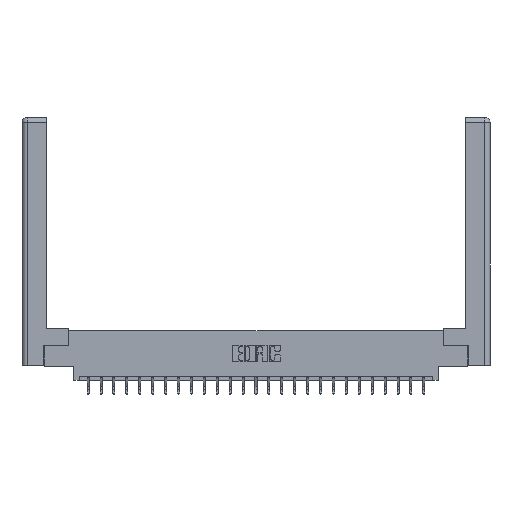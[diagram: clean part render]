
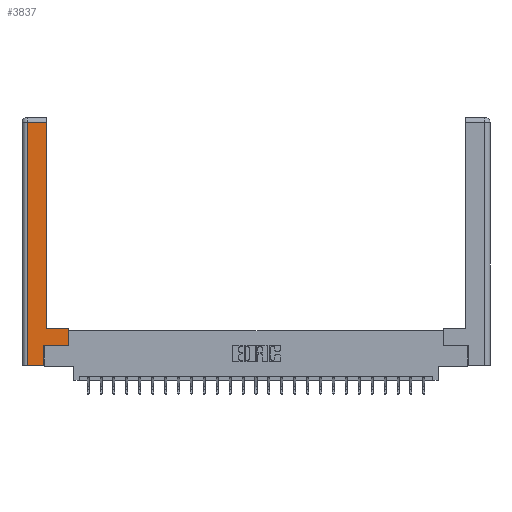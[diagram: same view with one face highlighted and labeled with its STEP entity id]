
A CAD part, top view. The second image highlights one B-rep face of the part: STEP entity #3837.
In plain terms, the highlighted planar face has unit normal (0, 0, 1).
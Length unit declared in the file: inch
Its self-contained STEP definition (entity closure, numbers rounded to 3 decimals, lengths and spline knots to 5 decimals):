
#94 = CARTESIAN_POINT ( 'NONE',  ( 0.295, 0.45, 0. ) ) ;
#168 = EDGE_LOOP ( 'NONE', ( #11904, #22617, #9253, #5354, #22514, #23321, #8111, #20060 ) ) ;
#1802 = CARTESIAN_POINT ( 'NONE',  ( 0.0615, 0., 0. ) ) ;
#2093 = FACE_OUTER_BOUND ( 'NONE', #168, .T. ) ;
#2310 = DIRECTION ( 'NONE',  ( 0., -1., 0. ) ) ;
#2415 = DIRECTION ( 'NONE',  ( 0., 1., 0. ) ) ;
#2947 = LINE ( 'NONE', #94, #7948 ) ;
#2972 = VECTOR ( 'NONE', #21944, 39.37008 ) ;
#3542 = VERTEX_POINT ( 'NONE', #5979 ) ;
#3837 = ADVANCED_FACE ( 'NONE', ( #2093 ), #12183, .F. ) ;
#4203 = LINE ( 'NONE', #12570, #6073 ) ;
#4324 = LINE ( 'NONE', #15668, #4620 ) ;
#4620 = VECTOR ( 'NONE', #9841, 39.37008 ) ;
#5225 = LINE ( 'NONE', #15964, #25583 ) ;
#5354 = ORIENTED_EDGE ( 'NONE', *, *, #21883, .T. ) ;
#5979 = CARTESIAN_POINT ( 'NONE',  ( 0.565, 0.45, 0. ) ) ;
#6031 = EDGE_CURVE ( 'NONE', #15035, #3542, #18403, .T. ) ;
#6073 = VECTOR ( 'NONE', #25053, 39.37008 ) ;
#6097 = DIRECTION ( 'NONE',  ( 0., 0., -1. ) ) ;
#6559 = CARTESIAN_POINT ( 'NONE',  ( 0.0615, 2.94, 0. ) ) ;
#7174 = VECTOR ( 'NONE', #2310, 39.37008 ) ;
#7285 = CARTESIAN_POINT ( 'NONE',  ( 0.295, 0.45, 0. ) ) ;
#7483 = CARTESIAN_POINT ( 'NONE',  ( 0.295, 2.94, 0. ) ) ;
#7785 = CARTESIAN_POINT ( 'NONE',  ( 0.565, 0.245, 0. ) ) ;
#7948 = VECTOR ( 'NONE', #22018, 39.37008 ) ;
#8111 = ORIENTED_EDGE ( 'NONE', *, *, #6031, .T. ) ;
#8415 = DIRECTION ( 'NONE',  ( -1., 0., 0. ) ) ;
#9169 = EDGE_CURVE ( 'NONE', #3542, #12504, #2947, .T. ) ;
#9253 = ORIENTED_EDGE ( 'NONE', *, *, #20976, .T. ) ;
#9328 = VECTOR ( 'NONE', #2415, 39.37008 ) ;
#9619 = CARTESIAN_POINT ( 'NONE',  ( 0.0615, 2.94, 0. ) ) ;
#9841 = DIRECTION ( 'NONE',  ( 0., 1., 0. ) ) ;
#10779 = CARTESIAN_POINT ( 'NONE',  ( 0.265, 0.245, 0. ) ) ;
#11264 = VECTOR ( 'NONE', #15727, 39.37008 ) ;
#11442 = CARTESIAN_POINT ( 'NONE',  ( 0.565, 0.245, 0. ) ) ;
#11863 = EDGE_CURVE ( 'NONE', #19201, #24317, #17455, .T. ) ;
#11904 = ORIENTED_EDGE ( 'NONE', *, *, #16731, .T. ) ;
#12183 = PLANE ( 'NONE',  #22511 ) ;
#12315 = CARTESIAN_POINT ( 'NONE',  ( 0.565, 0.45, 0. ) ) ;
#12369 = CARTESIAN_POINT ( 'NONE',  ( 0., 0., 0. ) ) ;
#12504 = VERTEX_POINT ( 'NONE', #7285 ) ;
#12570 = CARTESIAN_POINT ( 'NONE',  ( 0.295, 3., 0. ) ) ;
#14112 = EDGE_CURVE ( 'NONE', #19523, #18024, #4324, .T. ) ;
#15035 = VERTEX_POINT ( 'NONE', #11442 ) ;
#15098 = CARTESIAN_POINT ( 'NONE',  ( 0.265, 0., 0. ) ) ;
#15668 = CARTESIAN_POINT ( 'NONE',  ( 0.265, 0.245, 0. ) ) ;
#15727 = DIRECTION ( 'NONE',  ( -1., 0., 0. ) ) ;
#15964 = CARTESIAN_POINT ( 'NONE',  ( 0.265, 0., 0. ) ) ;
#16731 = EDGE_CURVE ( 'NONE', #12504, #19201, #4203, .T. ) ;
#17455 = LINE ( 'NONE', #9619, #11264 ) ;
#18024 = VERTEX_POINT ( 'NONE', #10779 ) ;
#18403 = LINE ( 'NONE', #12315, #9328 ) ;
#19201 = VERTEX_POINT ( 'NONE', #7483 ) ;
#19523 = VERTEX_POINT ( 'NONE', #15098 ) ;
#20060 = ORIENTED_EDGE ( 'NONE', *, *, #9169, .T. ) ;
#20976 = EDGE_CURVE ( 'NONE', #24317, #21808, #21552, .T. ) ;
#21552 = LINE ( 'NONE', #24078, #7174 ) ;
#21808 = VERTEX_POINT ( 'NONE', #1802 ) ;
#21883 = EDGE_CURVE ( 'NONE', #21808, #19523, #5225, .T. ) ;
#21944 = DIRECTION ( 'NONE',  ( 1., 0., 0. ) ) ;
#22018 = DIRECTION ( 'NONE',  ( -1., 0., 0. ) ) ;
#22511 = AXIS2_PLACEMENT_3D ( 'NONE', #12369, #6097, #8415 ) ;
#22514 = ORIENTED_EDGE ( 'NONE', *, *, #14112, .T. ) ;
#22617 = ORIENTED_EDGE ( 'NONE', *, *, #11863, .T. ) ;
#23321 = ORIENTED_EDGE ( 'NONE', *, *, #23819, .T. ) ;
#23532 = DIRECTION ( 'NONE',  ( 1., 0., 0. ) ) ;
#23819 = EDGE_CURVE ( 'NONE', #18024, #15035, #24247, .T. ) ;
#24078 = CARTESIAN_POINT ( 'NONE',  ( 0.0615, 0., 0. ) ) ;
#24247 = LINE ( 'NONE', #7785, #2972 ) ;
#24317 = VERTEX_POINT ( 'NONE', #6559 ) ;
#25053 = DIRECTION ( 'NONE',  ( 0., 1., 0. ) ) ;
#25583 = VECTOR ( 'NONE', #23532, 39.37008 ) ;
